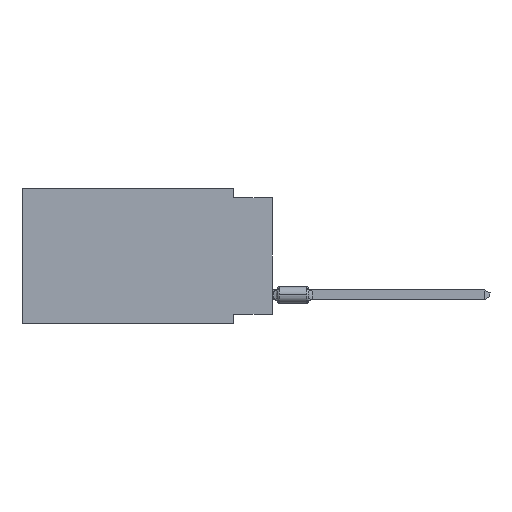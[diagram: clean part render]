
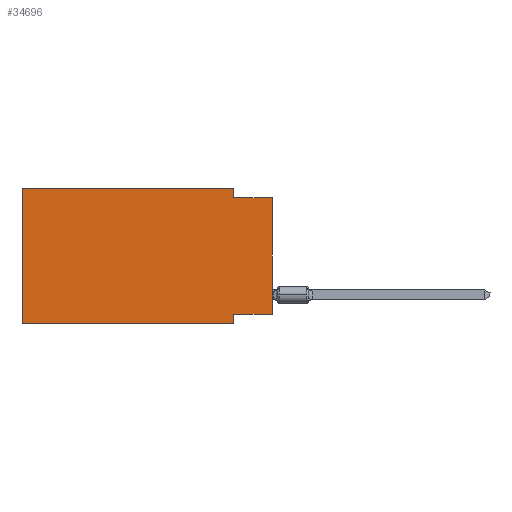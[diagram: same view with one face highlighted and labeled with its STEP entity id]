
A CAD part, left-side view. The second image highlights one B-rep face of the part: STEP entity #34696.
In plain terms, the highlighted planar face has unit normal (-1, 0, 0).
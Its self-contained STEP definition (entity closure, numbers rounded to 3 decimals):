
#1733 = CARTESIAN_POINT ( 'NONE',  ( 0., 0., -8.255 ) ) ;
#2370 = CARTESIAN_POINT ( 'NONE',  ( 0., 16.383, 0. ) ) ;
#3500 = LINE ( 'NONE', #37493, #34314 ) ;
#3781 = DIRECTION ( 'NONE',  ( 0., -1., 0. ) ) ;
#7596 = VECTOR ( 'NONE', #3781, 1000. ) ;
#8408 = DIRECTION ( 'NONE',  ( 0., 0., -1. ) ) ;
#10469 = CARTESIAN_POINT ( 'NONE',  ( 0., 16.383, -8.89 ) ) ;
#14123 = VECTOR ( 'NONE', #86453, 1000. ) ;
#18199 = AXIS2_PLACEMENT_3D ( 'NONE', #49159, #24595, #8408 ) ;
#19311 = EDGE_CURVE ( 'NONE', #27657, #50518, #93701, .T. ) ;
#23397 = DIRECTION ( 'NONE',  ( 0., 0., -1. ) ) ;
#24100 = VECTOR ( 'NONE', #76168, 1000. ) ;
#24274 = VERTEX_POINT ( 'NONE', #78142 ) ;
#24595 = DIRECTION ( 'NONE',  ( 1., 0., 0. ) ) ;
#24872 = DIRECTION ( 'NONE',  ( 0., 0., -1. ) ) ;
#26888 = ORIENTED_EDGE ( 'NONE', *, *, #49914, .T. ) ;
#26926 = CARTESIAN_POINT ( 'NONE',  ( 0., 2.54, -0.635 ) ) ;
#27657 = VERTEX_POINT ( 'NONE', #1733 ) ;
#29447 = LINE ( 'NONE', #48394, #29960 ) ;
#29960 = VECTOR ( 'NONE', #105844, 1000. ) ;
#31865 = VECTOR ( 'NONE', #68166, 1000. ) ;
#32972 = PLANE ( 'NONE',  #18199 ) ;
#34314 = VECTOR ( 'NONE', #71508, 1000. ) ;
#34319 = CARTESIAN_POINT ( 'NONE',  ( 0., 16.383, 0. ) ) ;
#34376 = ORIENTED_EDGE ( 'NONE', *, *, #45321, .F. ) ;
#34696 = ADVANCED_FACE ( 'NONE', ( #100986 ), #32972, .F. ) ;
#37493 = CARTESIAN_POINT ( 'NONE',  ( 0., 0., 0. ) ) ;
#42151 = LINE ( 'NONE', #34319, #24100 ) ;
#43485 = EDGE_LOOP ( 'NONE', ( #26888, #96747, #34376, #52879, #106851, #66980, #43641, #76101 ) ) ;
#43641 = ORIENTED_EDGE ( 'NONE', *, *, #104266, .F. ) ;
#45321 = EDGE_CURVE ( 'NONE', #58915, #108629, #99066, .T. ) ;
#48087 = CARTESIAN_POINT ( 'NONE',  ( 0., 2.54, -8.89 ) ) ;
#48394 = CARTESIAN_POINT ( 'NONE',  ( 0., 0., -0.635 ) ) ;
#49159 = CARTESIAN_POINT ( 'NONE',  ( 0., 16.383, 0. ) ) ;
#49914 = EDGE_CURVE ( 'NONE', #27657, #65442, #3500, .T. ) ;
#50113 = EDGE_CURVE ( 'NONE', #90484, #91244, #96862, .T. ) ;
#50518 = VERTEX_POINT ( 'NONE', #53813 ) ;
#52879 = ORIENTED_EDGE ( 'NONE', *, *, #68000, .F. ) ;
#53813 = CARTESIAN_POINT ( 'NONE',  ( 0., 2.54, -8.255 ) ) ;
#57244 = CARTESIAN_POINT ( 'NONE',  ( 0., 2.54, 0. ) ) ;
#58915 = VERTEX_POINT ( 'NONE', #94992 ) ;
#60809 = CARTESIAN_POINT ( 'NONE',  ( 0., 0., -8.255 ) ) ;
#62146 = EDGE_CURVE ( 'NONE', #108629, #65442, #29447, .T. ) ;
#65442 = VERTEX_POINT ( 'NONE', #74378 ) ;
#66980 = ORIENTED_EDGE ( 'NONE', *, *, #50113, .T. ) ;
#67495 = VECTOR ( 'NONE', #24872, 1000. ) ;
#68000 = EDGE_CURVE ( 'NONE', #24274, #58915, #42151, .T. ) ;
#68166 = DIRECTION ( 'NONE',  ( 0., 0., 1. ) ) ;
#71508 = DIRECTION ( 'NONE',  ( 0., 0., 1. ) ) ;
#71671 = VECTOR ( 'NONE', #23397, 1000. ) ;
#74378 = CARTESIAN_POINT ( 'NONE',  ( 0., 0., -0.635 ) ) ;
#76101 = ORIENTED_EDGE ( 'NONE', *, *, #19311, .F. ) ;
#76168 = DIRECTION ( 'NONE',  ( 0., -1., 0. ) ) ;
#78142 = CARTESIAN_POINT ( 'NONE',  ( 0., 16.383, 0. ) ) ;
#78753 = LINE ( 'NONE', #2370, #31865 ) ;
#82485 = CARTESIAN_POINT ( 'NONE',  ( 0., 16.383, -8.89 ) ) ;
#86453 = DIRECTION ( 'NONE',  ( 0., 1., 0. ) ) ;
#90484 = VERTEX_POINT ( 'NONE', #82485 ) ;
#91244 = VERTEX_POINT ( 'NONE', #48087 ) ;
#93701 = LINE ( 'NONE', #60809, #14123 ) ;
#94112 = EDGE_CURVE ( 'NONE', #90484, #24274, #78753, .T. ) ;
#94992 = CARTESIAN_POINT ( 'NONE',  ( 0., 2.54, 0. ) ) ;
#96747 = ORIENTED_EDGE ( 'NONE', *, *, #62146, .F. ) ;
#96862 = LINE ( 'NONE', #10469, #7596 ) ;
#99066 = LINE ( 'NONE', #57244, #67495 ) ;
#100986 = FACE_OUTER_BOUND ( 'NONE', #43485, .T. ) ;
#104266 = EDGE_CURVE ( 'NONE', #50518, #91244, #108690, .T. ) ;
#105844 = DIRECTION ( 'NONE',  ( 0., -1., 0. ) ) ;
#106851 = ORIENTED_EDGE ( 'NONE', *, *, #94112, .F. ) ;
#108144 = CARTESIAN_POINT ( 'NONE',  ( 0., 2.54, -8.89 ) ) ;
#108629 = VERTEX_POINT ( 'NONE', #26926 ) ;
#108690 = LINE ( 'NONE', #108144, #71671 ) ;
